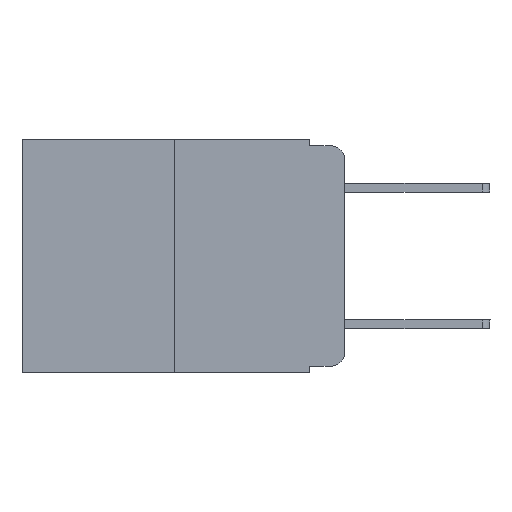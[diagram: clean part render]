
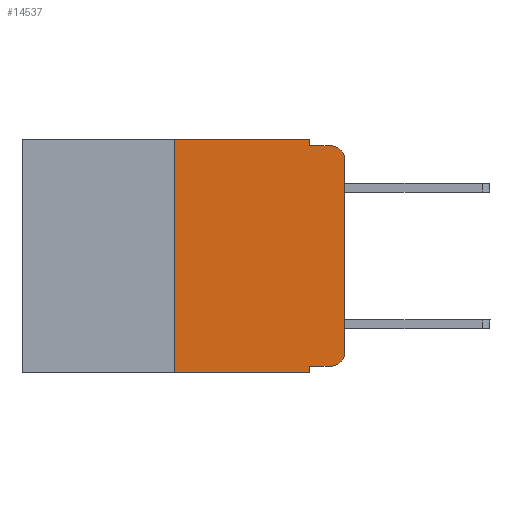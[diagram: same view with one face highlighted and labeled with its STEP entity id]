
A CAD part, left-side view. The second image highlights one B-rep face of the part: STEP entity #14537.
In plain terms, the highlighted planar face has unit normal (-1, 0, 0).
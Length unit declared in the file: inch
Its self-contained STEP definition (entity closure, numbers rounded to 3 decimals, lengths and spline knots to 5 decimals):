
#80 = ORIENTED_EDGE ( 'NONE', *, *, #15468, .F. ) ;
#118 = VERTEX_POINT ( 'NONE', #17380 ) ;
#185 = CARTESIAN_POINT ( 'NONE',  ( 0., 0.051, -0.333 ) ) ;
#268 = EDGE_CURVE ( 'NONE', #14595, #14372, #5468, .T. ) ;
#404 = ORIENTED_EDGE ( 'NONE', *, *, #16067, .T. ) ;
#667 = VECTOR ( 'NONE', #6718, 39.37008 ) ;
#1328 = PLANE ( 'NONE',  #11336 ) ;
#1721 = CARTESIAN_POINT ( 'NONE',  ( 0., 0.25, -0.343 ) ) ;
#2025 = CARTESIAN_POINT ( 'NONE',  ( 0., 0.051, 0. ) ) ;
#2129 = VECTOR ( 'NONE', #10350, 39.37008 ) ;
#2387 = EDGE_CURVE ( 'NONE', #17195, #118, #9622, .T. ) ;
#2412 = CARTESIAN_POINT ( 'NONE',  ( 0., 0.473, -0.343 ) ) ;
#2619 = ORIENTED_EDGE ( 'NONE', *, *, #268, .T. ) ;
#2685 = ORIENTED_EDGE ( 'NONE', *, *, #6787, .T. ) ;
#2698 = CARTESIAN_POINT ( 'NONE',  ( 0., 0.473, 0. ) ) ;
#2798 = ORIENTED_EDGE ( 'NONE', *, *, #5760, .F. ) ;
#3283 = VECTOR ( 'NONE', #10118, 39.37008 ) ;
#3290 = VERTEX_POINT ( 'NONE', #6813 ) ;
#3301 = ORIENTED_EDGE ( 'NONE', *, *, #2387, .T. ) ;
#3396 = DIRECTION ( 'NONE',  ( 0., 0., -1. ) ) ;
#3589 = LINE ( 'NONE', #2025, #16980 ) ;
#3995 = ORIENTED_EDGE ( 'NONE', *, *, #16884, .T. ) ;
#4655 = ORIENTED_EDGE ( 'NONE', *, *, #8998, .F. ) ;
#5107 = CIRCLE ( 'NONE', #10386, 0.02 ) ;
#5146 = DIRECTION ( 'NONE',  ( -1., 0., 0. ) ) ;
#5468 = LINE ( 'NONE', #185, #10282 ) ;
#5760 = EDGE_CURVE ( 'NONE', #14595, #15048, #10796, .T. ) ;
#5770 = CARTESIAN_POINT ( 'NONE',  ( 0., 0., 0. ) ) ;
#5960 = VECTOR ( 'NONE', #9331, 39.37008 ) ;
#6202 = VECTOR ( 'NONE', #15232, 39.37008 ) ;
#6718 = DIRECTION ( 'NONE',  ( 0., -1., 0. ) ) ;
#6767 = LINE ( 'NONE', #8698, #3283 ) ;
#6787 = EDGE_CURVE ( 'NONE', #13556, #15048, #16712, .T. ) ;
#6813 = CARTESIAN_POINT ( 'NONE',  ( 0., 0.051, -0.01 ) ) ;
#7084 = DIRECTION ( 'NONE',  ( 0., -1., 0. ) ) ;
#7692 = CARTESIAN_POINT ( 'NONE',  ( 0., 0.02, -0.01 ) ) ;
#7934 = CARTESIAN_POINT ( 'NONE',  ( 0., 0.25, 0. ) ) ;
#8000 = DIRECTION ( 'NONE',  ( 0., 0., 1. ) ) ;
#8134 = EDGE_CURVE ( 'NONE', #3290, #13688, #6767, .T. ) ;
#8348 = DIRECTION ( 'NONE',  ( 0., 0., -1. ) ) ;
#8516 = AXIS2_PLACEMENT_3D ( 'NONE', #9305, #5146, #10730 ) ;
#8529 = VERTEX_POINT ( 'NONE', #12607 ) ;
#8698 = CARTESIAN_POINT ( 'NONE',  ( 0., 0.051, -0.01 ) ) ;
#8998 = EDGE_CURVE ( 'NONE', #13556, #8529, #12492, .T. ) ;
#9305 = CARTESIAN_POINT ( 'NONE',  ( 0., 0.02, -0.03 ) ) ;
#9331 = DIRECTION ( 'NONE',  ( 0., 0., -1. ) ) ;
#9462 = ORIENTED_EDGE ( 'NONE', *, *, #15733, .F. ) ;
#9622 = LINE ( 'NONE', #5770, #2129 ) ;
#10118 = DIRECTION ( 'NONE',  ( 0., -1., 0. ) ) ;
#10282 = VECTOR ( 'NONE', #7084, 39.37008 ) ;
#10350 = DIRECTION ( 'NONE',  ( 0., 0., 1. ) ) ;
#10363 = CARTESIAN_POINT ( 'NONE',  ( 0., 0.051, 0. ) ) ;
#10386 = AXIS2_PLACEMENT_3D ( 'NONE', #11713, #16186, #10559 ) ;
#10559 = DIRECTION ( 'NONE',  ( 0., 0., -1. ) ) ;
#10730 = DIRECTION ( 'NONE',  ( 0., 0., -1. ) ) ;
#10796 = LINE ( 'NONE', #16451, #5960 ) ;
#11031 = CARTESIAN_POINT ( 'NONE',  ( 0., 0.051, -0.343 ) ) ;
#11059 = EDGE_LOOP ( 'NONE', ( #3301, #3995, #16469, #80, #9462, #4655, #2685, #2798, #2619, #404 ) ) ;
#11336 = AXIS2_PLACEMENT_3D ( 'NONE', #2698, #12530, #8348 ) ;
#11390 = CARTESIAN_POINT ( 'NONE',  ( 0., 0.02, -0.333 ) ) ;
#11713 = CARTESIAN_POINT ( 'NONE',  ( 0., 0.02, -0.313 ) ) ;
#12492 = LINE ( 'NONE', #7934, #17932 ) ;
#12530 = DIRECTION ( 'NONE',  ( 1., 0., 0. ) ) ;
#12607 = CARTESIAN_POINT ( 'NONE',  ( 0., 0.25, 0. ) ) ;
#13556 = VERTEX_POINT ( 'NONE', #1721 ) ;
#13660 = CIRCLE ( 'NONE', #8516, 0.02 ) ;
#13688 = VERTEX_POINT ( 'NONE', #7692 ) ;
#13698 = LINE ( 'NONE', #13904, #6202 ) ;
#13904 = CARTESIAN_POINT ( 'NONE',  ( 0., 0.473, 0. ) ) ;
#13977 = FACE_OUTER_BOUND ( 'NONE', #11059, .T. ) ;
#14065 = CARTESIAN_POINT ( 'NONE',  ( 0., 0.051, -0.333 ) ) ;
#14104 = CARTESIAN_POINT ( 'NONE',  ( 0., 0., -0.313 ) ) ;
#14372 = VERTEX_POINT ( 'NONE', #11390 ) ;
#14537 = ADVANCED_FACE ( 'NONE', ( #13977 ), #1328, .F. ) ;
#14595 = VERTEX_POINT ( 'NONE', #14065 ) ;
#15048 = VERTEX_POINT ( 'NONE', #11031 ) ;
#15232 = DIRECTION ( 'NONE',  ( 0., -1., 0. ) ) ;
#15468 = EDGE_CURVE ( 'NONE', #16184, #3290, #3589, .T. ) ;
#15733 = EDGE_CURVE ( 'NONE', #8529, #16184, #13698, .T. ) ;
#16067 = EDGE_CURVE ( 'NONE', #14372, #17195, #5107, .T. ) ;
#16184 = VERTEX_POINT ( 'NONE', #10363 ) ;
#16186 = DIRECTION ( 'NONE',  ( -1., 0., 0. ) ) ;
#16451 = CARTESIAN_POINT ( 'NONE',  ( 0., 0.051, 0. ) ) ;
#16469 = ORIENTED_EDGE ( 'NONE', *, *, #8134, .F. ) ;
#16712 = LINE ( 'NONE', #2412, #667 ) ;
#16884 = EDGE_CURVE ( 'NONE', #118, #13688, #13660, .T. ) ;
#16980 = VECTOR ( 'NONE', #3396, 39.37008 ) ;
#17195 = VERTEX_POINT ( 'NONE', #14104 ) ;
#17380 = CARTESIAN_POINT ( 'NONE',  ( 0., 0., -0.03 ) ) ;
#17932 = VECTOR ( 'NONE', #8000, 39.37008 ) ;
